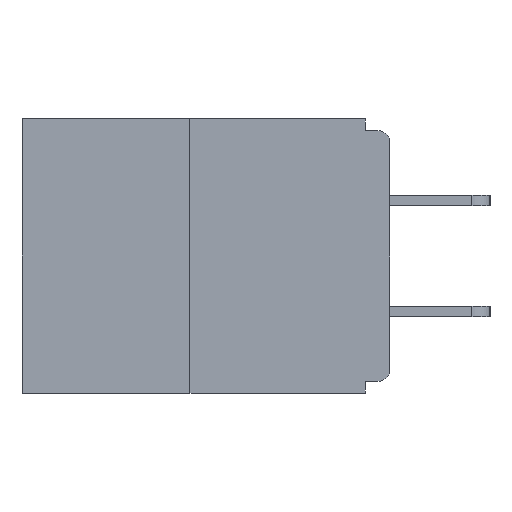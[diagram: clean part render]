
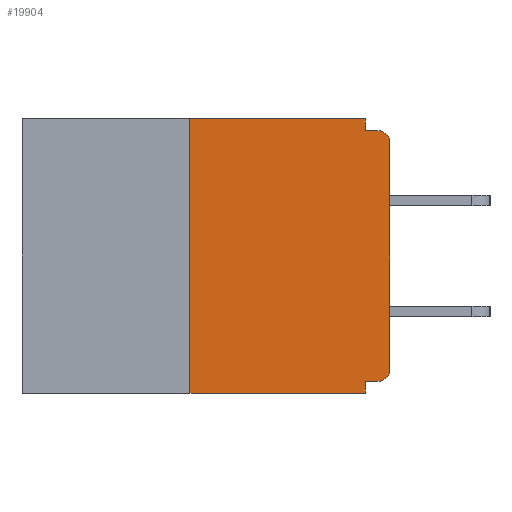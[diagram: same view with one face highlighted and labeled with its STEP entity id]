
A CAD part, left-side view. The second image highlights one B-rep face of the part: STEP entity #19904.
In plain terms, the highlighted planar face has unit normal (-1, 0, 0).
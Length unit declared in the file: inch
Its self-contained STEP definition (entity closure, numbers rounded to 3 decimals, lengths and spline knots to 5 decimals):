
#1373 = DIRECTION ( 'NONE',  ( 0., 0., -1. ) ) ;
#1865 = LINE ( 'NONE', #19897, #29277 ) ;
#2575 = DIRECTION ( 'NONE',  ( 1., 0., 0. ) ) ;
#3501 = EDGE_CURVE ( 'NONE', #29214, #23877, #13413, .T. ) ;
#3626 = CARTESIAN_POINT ( 'NONE',  ( 0., 0.031, 0. ) ) ;
#3653 = VECTOR ( 'NONE', #26997, 39.37008 ) ;
#4094 = VECTOR ( 'NONE', #22713, 39.37008 ) ;
#4344 = AXIS2_PLACEMENT_3D ( 'NONE', #23200, #16167, #14654 ) ;
#4468 = DIRECTION ( 'NONE',  ( 0., 0., 1. ) ) ;
#4528 = PLANE ( 'NONE',  #7942 ) ;
#5565 = CARTESIAN_POINT ( 'NONE',  ( 0., 0.25, 0. ) ) ;
#5581 = ORIENTED_EDGE ( 'NONE', *, *, #7939, .F. ) ;
#5758 = CIRCLE ( 'NONE', #4344, 0.015 ) ;
#6144 = EDGE_CURVE ( 'NONE', #25779, #23877, #24368, .T. ) ;
#6267 = LINE ( 'NONE', #24446, #26917 ) ;
#6572 = VERTEX_POINT ( 'NONE', #26286 ) ;
#6717 = ORIENTED_EDGE ( 'NONE', *, *, #18089, .F. ) ;
#7097 = EDGE_CURVE ( 'NONE', #23433, #6572, #8770, .T. ) ;
#7939 = EDGE_CURVE ( 'NONE', #6572, #19141, #17160, .T. ) ;
#7942 = AXIS2_PLACEMENT_3D ( 'NONE', #11061, #2575, #27467 ) ;
#7947 = ORIENTED_EDGE ( 'NONE', *, *, #7097, .F. ) ;
#8376 = EDGE_CURVE ( 'NONE', #13210, #9631, #9054, .T. ) ;
#8431 = VERTEX_POINT ( 'NONE', #22495 ) ;
#8475 = CARTESIAN_POINT ( 'NONE',  ( 0., 0., 0. ) ) ;
#8770 = LINE ( 'NONE', #17862, #9942 ) ;
#8959 = EDGE_CURVE ( 'NONE', #8431, #13210, #5758, .T. ) ;
#9054 = LINE ( 'NONE', #8475, #24775 ) ;
#9223 = CARTESIAN_POINT ( 'NONE',  ( 0., 0.031, -0.343 ) ) ;
#9631 = VERTEX_POINT ( 'NONE', #10140 ) ;
#9942 = VECTOR ( 'NONE', #19974, 39.37008 ) ;
#10140 = CARTESIAN_POINT ( 'NONE',  ( 0., 0., -0.03 ) ) ;
#10331 = ORIENTED_EDGE ( 'NONE', *, *, #20260, .F. ) ;
#11061 = CARTESIAN_POINT ( 'NONE',  ( 0., 0.46, 0. ) ) ;
#11314 = ORIENTED_EDGE ( 'NONE', *, *, #3501, .F. ) ;
#11457 = EDGE_CURVE ( 'NONE', #9631, #19643, #17584, .T. ) ;
#12264 = LINE ( 'NONE', #5565, #23062 ) ;
#12723 = CARTESIAN_POINT ( 'NONE',  ( 0., 0., -0.313 ) ) ;
#13210 = VERTEX_POINT ( 'NONE', #12723 ) ;
#13306 = AXIS2_PLACEMENT_3D ( 'NONE', #14651, #15083, #28368 ) ;
#13413 = LINE ( 'NONE', #9223, #3653 ) ;
#14581 = CARTESIAN_POINT ( 'NONE',  ( 0., 0.031, -0.343 ) ) ;
#14651 = CARTESIAN_POINT ( 'NONE',  ( 0., 0.015, -0.03 ) ) ;
#14654 = DIRECTION ( 'NONE',  ( 0., 0., -1. ) ) ;
#14751 = CARTESIAN_POINT ( 'NONE',  ( 0., 0.25, -0.343 ) ) ;
#15083 = DIRECTION ( 'NONE',  ( -1., 0., 0. ) ) ;
#15270 = DIRECTION ( 'NONE',  ( 0., -1., 0. ) ) ;
#16167 = DIRECTION ( 'NONE',  ( -1., 0., 0. ) ) ;
#17116 = VECTOR ( 'NONE', #1373, 39.37008 ) ;
#17160 = LINE ( 'NONE', #3626, #17116 ) ;
#17584 = CIRCLE ( 'NONE', #13306, 0.015 ) ;
#17862 = CARTESIAN_POINT ( 'NONE',  ( 0., 0.46, 0. ) ) ;
#18089 = EDGE_CURVE ( 'NONE', #8431, #29214, #6267, .T. ) ;
#18354 = FACE_OUTER_BOUND ( 'NONE', #23485, .T. ) ;
#19093 = CARTESIAN_POINT ( 'NONE',  ( 0., 0.25, 0. ) ) ;
#19141 = VERTEX_POINT ( 'NONE', #21707 ) ;
#19556 = DIRECTION ( 'NONE',  ( 0., 0., 1. ) ) ;
#19643 = VERTEX_POINT ( 'NONE', #23626 ) ;
#19894 = CARTESIAN_POINT ( 'NONE',  ( 0., 0.46, -0.343 ) ) ;
#19897 = CARTESIAN_POINT ( 'NONE',  ( 0., 0., -0.015 ) ) ;
#19904 = ADVANCED_FACE ( 'NONE', ( #18354 ), #4528, .F. ) ;
#19974 = DIRECTION ( 'NONE',  ( 0., -1., 0. ) ) ;
#20260 = EDGE_CURVE ( 'NONE', #25779, #23433, #12264, .T. ) ;
#20651 = ORIENTED_EDGE ( 'NONE', *, *, #6144, .T. ) ;
#21707 = CARTESIAN_POINT ( 'NONE',  ( 0., 0.031, -0.015 ) ) ;
#22217 = DIRECTION ( 'NONE',  ( 0., 1., 0. ) ) ;
#22495 = CARTESIAN_POINT ( 'NONE',  ( 0., 0.015, -0.328 ) ) ;
#22713 = DIRECTION ( 'NONE',  ( 0., -1., 0. ) ) ;
#22846 = EDGE_CURVE ( 'NONE', #19141, #19643, #1865, .T. ) ;
#23062 = VECTOR ( 'NONE', #19556, 39.37008 ) ;
#23200 = CARTESIAN_POINT ( 'NONE',  ( 0., 0.015, -0.313 ) ) ;
#23433 = VERTEX_POINT ( 'NONE', #19093 ) ;
#23485 = EDGE_LOOP ( 'NONE', ( #7947, #10331, #20651, #11314, #6717, #28666, #24918, #24084, #23551, #5581 ) ) ;
#23551 = ORIENTED_EDGE ( 'NONE', *, *, #22846, .F. ) ;
#23626 = CARTESIAN_POINT ( 'NONE',  ( 0., 0.015, -0.015 ) ) ;
#23877 = VERTEX_POINT ( 'NONE', #14581 ) ;
#24084 = ORIENTED_EDGE ( 'NONE', *, *, #11457, .T. ) ;
#24368 = LINE ( 'NONE', #19894, #4094 ) ;
#24446 = CARTESIAN_POINT ( 'NONE',  ( 0., 0., -0.328 ) ) ;
#24775 = VECTOR ( 'NONE', #4468, 39.37008 ) ;
#24918 = ORIENTED_EDGE ( 'NONE', *, *, #8376, .T. ) ;
#25779 = VERTEX_POINT ( 'NONE', #14751 ) ;
#26286 = CARTESIAN_POINT ( 'NONE',  ( 0., 0.031, 0. ) ) ;
#26917 = VECTOR ( 'NONE', #22217, 39.37008 ) ;
#26997 = DIRECTION ( 'NONE',  ( 0., 0., -1. ) ) ;
#27467 = DIRECTION ( 'NONE',  ( 0., 0., -1. ) ) ;
#28368 = DIRECTION ( 'NONE',  ( 0., 0., -1. ) ) ;
#28666 = ORIENTED_EDGE ( 'NONE', *, *, #8959, .T. ) ;
#28897 = CARTESIAN_POINT ( 'NONE',  ( 0., 0.031, -0.328 ) ) ;
#29214 = VERTEX_POINT ( 'NONE', #28897 ) ;
#29277 = VECTOR ( 'NONE', #15270, 39.37008 ) ;
